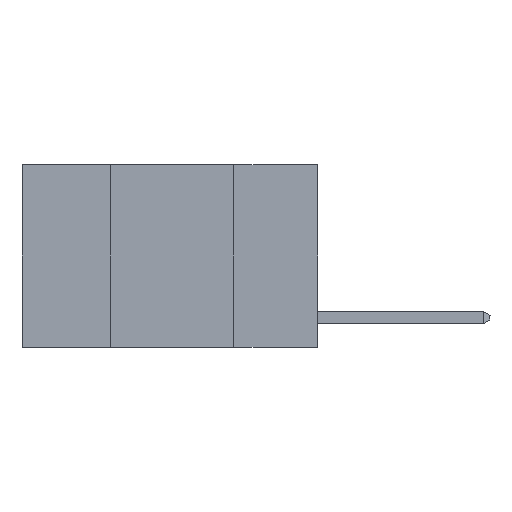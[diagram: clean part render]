
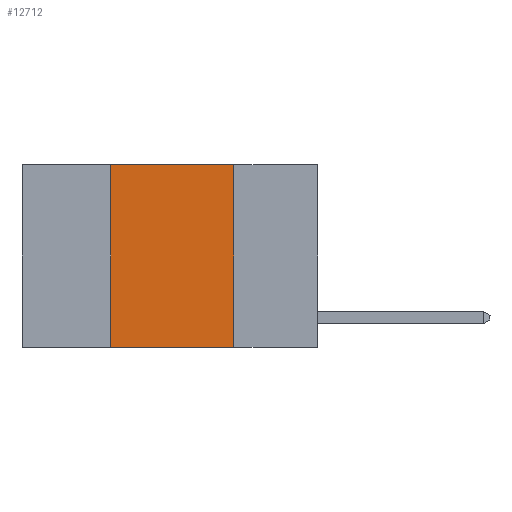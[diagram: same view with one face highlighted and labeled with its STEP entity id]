
A CAD part, left-side view. The second image highlights one B-rep face of the part: STEP entity #12712.
In plain terms, the highlighted planar face has unit normal (-1, 0, 0).
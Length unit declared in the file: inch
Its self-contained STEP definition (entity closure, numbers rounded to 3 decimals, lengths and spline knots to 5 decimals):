
#131 = EDGE_CURVE ( 'NONE', #8644, #12869, #16426, .T. ) ;
#148 = CARTESIAN_POINT ( 'NONE',  ( 0., 0.42, -0.37 ) ) ;
#401 = VECTOR ( 'NONE', #9975, 39.37008 ) ;
#435 = CARTESIAN_POINT ( 'NONE',  ( 0., 0.17, -0.37 ) ) ;
#2148 = PLANE ( 'NONE',  #12835 ) ;
#2567 = VECTOR ( 'NONE', #9064, 39.37008 ) ;
#3564 = EDGE_LOOP ( 'NONE', ( #6564, #5710, #12526, #5635 ) ) ;
#4418 = DIRECTION ( 'NONE',  ( 1., 0., 0. ) ) ;
#5277 = VECTOR ( 'NONE', #16285, 39.37008 ) ;
#5352 = CARTESIAN_POINT ( 'NONE',  ( 0., 0.6, -0.37 ) ) ;
#5635 = ORIENTED_EDGE ( 'NONE', *, *, #12931, .T. ) ;
#5710 = ORIENTED_EDGE ( 'NONE', *, *, #131, .F. ) ;
#5955 = LINE ( 'NONE', #11118, #5277 ) ;
#6254 = EDGE_CURVE ( 'NONE', #6362, #8644, #12501, .T. ) ;
#6362 = VERTEX_POINT ( 'NONE', #148 ) ;
#6564 = ORIENTED_EDGE ( 'NONE', *, *, #12782, .F. ) ;
#8236 = DIRECTION ( 'NONE',  ( 0., 0., -1. ) ) ;
#8448 = CARTESIAN_POINT ( 'NONE',  ( 0., 0.42, 0. ) ) ;
#8565 = VERTEX_POINT ( 'NONE', #435 ) ;
#8644 = VERTEX_POINT ( 'NONE', #8448 ) ;
#9064 = DIRECTION ( 'NONE',  ( 0., -1., 0. ) ) ;
#9407 = LINE ( 'NONE', #5352, #2567 ) ;
#9495 = FACE_OUTER_BOUND ( 'NONE', #3564, .T. ) ;
#9975 = DIRECTION ( 'NONE',  ( 0., 0., 1. ) ) ;
#11118 = CARTESIAN_POINT ( 'NONE',  ( 0., 0.17, 0. ) ) ;
#11289 = CARTESIAN_POINT ( 'NONE',  ( 0., 0.17, 0. ) ) ;
#12352 = CARTESIAN_POINT ( 'NONE',  ( 0., 0.6, 0. ) ) ;
#12501 = LINE ( 'NONE', #15393, #401 ) ;
#12526 = ORIENTED_EDGE ( 'NONE', *, *, #6254, .F. ) ;
#12712 = ADVANCED_FACE ( 'NONE', ( #9495 ), #2148, .F. ) ;
#12782 = EDGE_CURVE ( 'NONE', #12869, #8565, #5955, .T. ) ;
#12835 = AXIS2_PLACEMENT_3D ( 'NONE', #14835, #4418, #8236 ) ;
#12869 = VERTEX_POINT ( 'NONE', #11289 ) ;
#12931 = EDGE_CURVE ( 'NONE', #6362, #8565, #9407, .T. ) ;
#14835 = CARTESIAN_POINT ( 'NONE',  ( 0., 0.6, 0. ) ) ;
#15195 = VECTOR ( 'NONE', #16090, 39.37008 ) ;
#15393 = CARTESIAN_POINT ( 'NONE',  ( 0., 0.42, 0. ) ) ;
#16090 = DIRECTION ( 'NONE',  ( 0., -1., 0. ) ) ;
#16285 = DIRECTION ( 'NONE',  ( 0., 0., -1. ) ) ;
#16426 = LINE ( 'NONE', #12352, #15195 ) ;
